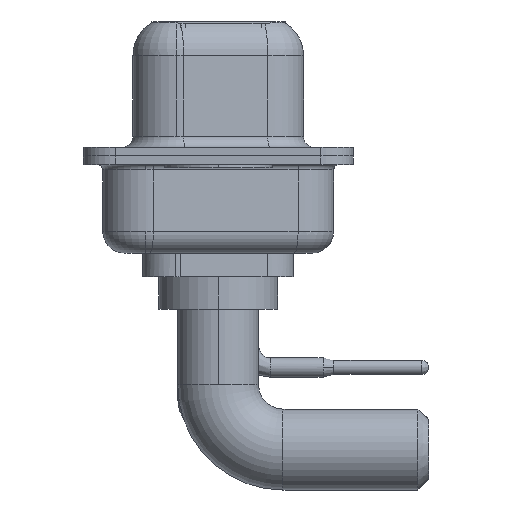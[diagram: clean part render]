
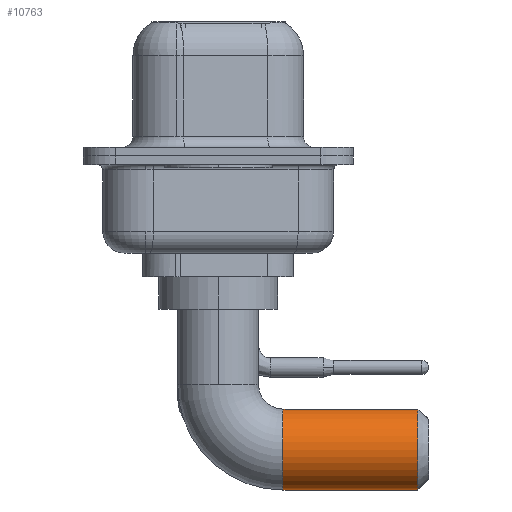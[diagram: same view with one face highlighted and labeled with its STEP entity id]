
A CAD part, left-side view. The second image highlights one B-rep face of the part: STEP entity #10763.
In plain terms, the highlighted cylindrical face has radius 1.875 mm (diameter 3.75 mm), a partial arc.
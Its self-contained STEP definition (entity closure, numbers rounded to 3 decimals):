
#217 = LINE ( 'NONE', #7299, #11116 ) ;
#2449 = CARTESIAN_POINT ( 'NONE',  ( 0., -3., -4.625 ) ) ;
#2480 = CARTESIAN_POINT ( 'NONE',  ( 0., -3., -6.5 ) ) ;
#3145 = CARTESIAN_POINT ( 'NONE',  ( 0., -3., -6.5 ) ) ;
#3619 = VERTEX_POINT ( 'NONE', #13303 ) ;
#7174 = EDGE_CURVE ( 'NONE', #7639, #3619, #21573, .T. ) ;
#7299 = CARTESIAN_POINT ( 'NONE',  ( 0., -3., -8.375 ) ) ;
#7639 = VERTEX_POINT ( 'NONE', #2449 ) ;
#7661 = CARTESIAN_POINT ( 'NONE',  ( 0., -3., -4.625 ) ) ;
#7787 = ORIENTED_EDGE ( 'NONE', *, *, #7174, .T. ) ;
#7958 = AXIS2_PLACEMENT_3D ( 'NONE', #2480, #21090, #18876 ) ;
#7999 = ORIENTED_EDGE ( 'NONE', *, *, #20634, .F. ) ;
#8274 = AXIS2_PLACEMENT_3D ( 'NONE', #16172, #13485, #9415 ) ;
#8450 = EDGE_LOOP ( 'NONE', ( #7999, #7787, #11897, #8734 ) ) ;
#8734 = ORIENTED_EDGE ( 'NONE', *, *, #14013, .T. ) ;
#9182 = DIRECTION ( 'NONE',  ( 0., -1., 0. ) ) ;
#9269 = EDGE_CURVE ( 'NONE', #3619, #18088, #217, .T. ) ;
#9415 = DIRECTION ( 'NONE',  ( 0., 0., -1. ) ) ;
#10763 = ADVANCED_FACE ( 'NONE', ( #22482 ), #18862, .T. ) ;
#11116 = VECTOR ( 'NONE', #21523, 1000. ) ;
#11897 = ORIENTED_EDGE ( 'NONE', *, *, #9269, .T. ) ;
#12567 = LINE ( 'NONE', #7661, #15664 ) ;
#13303 = CARTESIAN_POINT ( 'NONE',  ( 0., -3., -8.375 ) ) ;
#13485 = DIRECTION ( 'NONE',  ( 0., 1., 0. ) ) ;
#14013 = EDGE_CURVE ( 'NONE', #18088, #23008, #14591, .T. ) ;
#14591 = CIRCLE ( 'NONE', #8274, 1.875 ) ;
#15140 = DIRECTION ( 'NONE',  ( 0., -1., 0. ) ) ;
#15664 = VECTOR ( 'NONE', #9182, 1000. ) ;
#16172 = CARTESIAN_POINT ( 'NONE',  ( 0., -9.25, -6.5 ) ) ;
#16369 = AXIS2_PLACEMENT_3D ( 'NONE', #3145, #15140, #17224 ) ;
#17224 = DIRECTION ( 'NONE',  ( 0., 0., -1. ) ) ;
#18088 = VERTEX_POINT ( 'NONE', #19197 ) ;
#18862 = CYLINDRICAL_SURFACE ( 'NONE', #16369, 1.875 ) ;
#18876 = DIRECTION ( 'NONE',  ( -1., 0., 0. ) ) ;
#19197 = CARTESIAN_POINT ( 'NONE',  ( 0., -9.25, -8.375 ) ) ;
#19734 = CARTESIAN_POINT ( 'NONE',  ( 0., -9.25, -4.625 ) ) ;
#20634 = EDGE_CURVE ( 'NONE', #7639, #23008, #12567, .T. ) ;
#21090 = DIRECTION ( 'NONE',  ( 0., -1., 0. ) ) ;
#21523 = DIRECTION ( 'NONE',  ( 0., -1., 0. ) ) ;
#21573 = CIRCLE ( 'NONE', #7958, 1.875 ) ;
#22482 = FACE_OUTER_BOUND ( 'NONE', #8450, .T. ) ;
#23008 = VERTEX_POINT ( 'NONE', #19734 ) ;
